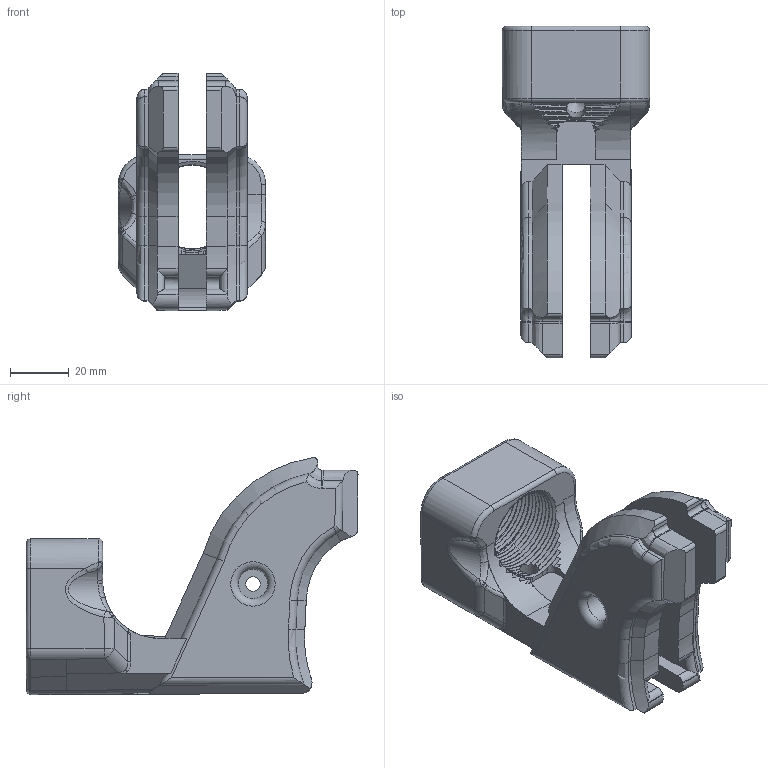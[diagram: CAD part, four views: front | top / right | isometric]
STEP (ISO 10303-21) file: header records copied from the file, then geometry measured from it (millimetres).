
FILE_DESCRIPTION(/* description */ (''),/* implementation_level */ '2;1');
FILE_NAME(/* name */ 'HRR - Buffer Tube + Grip Adapter Redux v3.step',/* time_stamp */ '2020-03-16T00:38:02-04:00',/* author */ (''),/* organization */ (''),/* preprocessor_version */ 'ST-DEVELOPER v18',/* originating_system */ 'Autodesk Translation Framework v8.12.0.6',/* authorisation */ '');
FILE_SCHEMA (('AUTOMOTIVE_DESIGN { 1 0 10303 214 3 1 1 }'));
Length unit declared in the file: millimetre
Products named in the file (1): HRR - Buffer Tube + Grip Adapter Redux
Bounding box: 50 x 112.77 x 80.55 mm (x, y, z)
Volume: 140786.6 mm3; surface area: 34443.6 mm2
Topology: 1 solids, 1 shells, 307 faces, 830 edges, 523 vertices
Faces by surface type: cylinder 125, plane 85, bspline 63, torus 26, cone 7, sphere 1
Full cylindrical faces by diameter (mm): 4.39 x2, 5 x2, 6.477 x1, 10 x1, 10.075 x1, 28.575 x15
Entity records: 26220 total; most frequent: CARTESIAN_POINT 19173, ORIENTED_EDGE 1654, DIRECTION 1216, EDGE_CURVE 827, VERTEX_POINT 523, AXIS2_PLACEMENT_3D 468, B_SPLINE_CURVE_WITH_KNOTS 315, EDGE_LOOP 314
